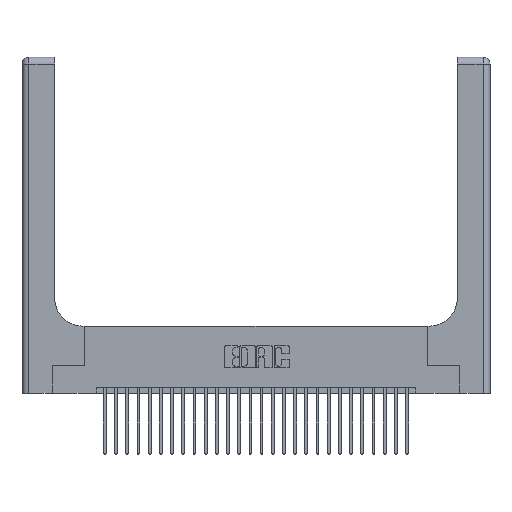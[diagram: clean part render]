
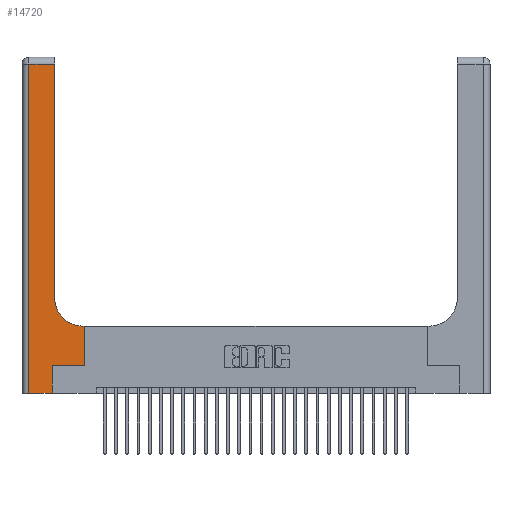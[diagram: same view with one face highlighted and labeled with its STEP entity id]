
A CAD part, top view. The second image highlights one B-rep face of the part: STEP entity #14720.
In plain terms, the highlighted planar face has unit normal (0, 0, 1).
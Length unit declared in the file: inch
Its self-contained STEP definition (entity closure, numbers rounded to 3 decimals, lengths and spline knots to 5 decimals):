
#814 = EDGE_CURVE ( 'NONE', #4730, #16422, #15518, .T. ) ;
#1194 = ORIENTED_EDGE ( 'NONE', *, *, #24007, .T. ) ;
#1438 = VERTEX_POINT ( 'NONE', #7639 ) ;
#1827 = VECTOR ( 'NONE', #13292, 39.37008 ) ;
#3280 = VECTOR ( 'NONE', #25573, 39.37008 ) ;
#4053 = VECTOR ( 'NONE', #12388, 39.37008 ) ;
#4461 = CARTESIAN_POINT ( 'NONE',  ( 0.06, 3., 0.37 ) ) ;
#4730 = VERTEX_POINT ( 'NONE', #5925 ) ;
#4941 = CARTESIAN_POINT ( 'NONE',  ( 0.06, 0., 0.37 ) ) ;
#5925 = CARTESIAN_POINT ( 'NONE',  ( 0.269, 0., 0.37 ) ) ;
#5981 = CIRCLE ( 'NONE', #23748, 0.25 ) ;
#6549 = LINE ( 'NONE', #12526, #28282 ) ;
#7168 = DIRECTION ( 'NONE',  ( 0., 0., -1. ) ) ;
#7337 = CARTESIAN_POINT ( 'NONE',  ( 0.2915, 2.94, 0.37 ) ) ;
#7361 = PLANE ( 'NONE',  #12674 ) ;
#7451 = VERTEX_POINT ( 'NONE', #16705 ) ;
#7639 = CARTESIAN_POINT ( 'NONE',  ( 0.06, 2.94, 0.37 ) ) ;
#8438 = ORIENTED_EDGE ( 'NONE', *, *, #15422, .T. ) ;
#8717 = CARTESIAN_POINT ( 'NONE',  ( 0.5415, 0.6, 0.37 ) ) ;
#10127 = CARTESIAN_POINT ( 'NONE',  ( 0.5585, 0.25, 0.37 ) ) ;
#10385 = CARTESIAN_POINT ( 'NONE',  ( 0.2915, 0.6, 0.37 ) ) ;
#10492 = CARTESIAN_POINT ( 'NONE',  ( 0.5585, 0.25, 0.37 ) ) ;
#11010 = CARTESIAN_POINT ( 'NONE',  ( 0.269, 0.25, 0.37 ) ) ;
#11692 = LINE ( 'NONE', #4461, #16961 ) ;
#11914 = CARTESIAN_POINT ( 'NONE',  ( 0., 3., 0.37 ) ) ;
#12181 = CARTESIAN_POINT ( 'NONE',  ( 0., 0., 0.37 ) ) ;
#12295 = VERTEX_POINT ( 'NONE', #8717 ) ;
#12388 = DIRECTION ( 'NONE',  ( 0., 1., 0. ) ) ;
#12506 = ORIENTED_EDGE ( 'NONE', *, *, #28689, .T. ) ;
#12526 = CARTESIAN_POINT ( 'NONE',  ( 0.2915, 3., 0.37 ) ) ;
#12674 = AXIS2_PLACEMENT_3D ( 'NONE', #11914, #27552, #14192 ) ;
#13132 = VERTEX_POINT ( 'NONE', #7337 ) ;
#13292 = DIRECTION ( 'NONE',  ( 1., 0., 0. ) ) ;
#13772 = ORIENTED_EDGE ( 'NONE', *, *, #25143, .T. ) ;
#13890 = LINE ( 'NONE', #12181, #3280 ) ;
#13974 = VERTEX_POINT ( 'NONE', #10492 ) ;
#14155 = CARTESIAN_POINT ( 'NONE',  ( 0., 2.94, 0.37 ) ) ;
#14192 = DIRECTION ( 'NONE',  ( -1., 0., 0. ) ) ;
#14537 = LINE ( 'NONE', #11010, #1827 ) ;
#14594 = LINE ( 'NONE', #14155, #25773 ) ;
#14720 = ADVANCED_FACE ( 'NONE', ( #25456 ), #7361, .F. ) ;
#14789 = DIRECTION ( 'NONE',  ( 0., 1., 0. ) ) ;
#15374 = EDGE_CURVE ( 'NONE', #13132, #1438, #14594, .T. ) ;
#15384 = VERTEX_POINT ( 'NONE', #23232 ) ;
#15422 = EDGE_CURVE ( 'NONE', #18927, #4730, #13890, .T. ) ;
#15518 = LINE ( 'NONE', #16725, #27376 ) ;
#16422 = VERTEX_POINT ( 'NONE', #17893 ) ;
#16705 = CARTESIAN_POINT ( 'NONE',  ( 0.2915, 0.85, 0.37 ) ) ;
#16725 = CARTESIAN_POINT ( 'NONE',  ( 0.269, 0., 0.37 ) ) ;
#16821 = ORIENTED_EDGE ( 'NONE', *, *, #15374, .T. ) ;
#16917 = ORIENTED_EDGE ( 'NONE', *, *, #27693, .T. ) ;
#16961 = VECTOR ( 'NONE', #17948, 39.37008 ) ;
#17143 = DIRECTION ( 'NONE',  ( -1., 0., 0. ) ) ;
#17893 = CARTESIAN_POINT ( 'NONE',  ( 0.269, 0.25, 0.37 ) ) ;
#17948 = DIRECTION ( 'NONE',  ( 0., -1., 0. ) ) ;
#18627 = DIRECTION ( 'NONE',  ( -1., 0., 0. ) ) ;
#18927 = VERTEX_POINT ( 'NONE', #4941 ) ;
#20297 = VECTOR ( 'NONE', #17143, 39.37008 ) ;
#20626 = CARTESIAN_POINT ( 'NONE',  ( 0.5415, 0.85, 0.37 ) ) ;
#21302 = ORIENTED_EDGE ( 'NONE', *, *, #26516, .T. ) ;
#21704 = LINE ( 'NONE', #10385, #20297 ) ;
#22689 = LINE ( 'NONE', #10127, #4053 ) ;
#22880 = DIRECTION ( 'NONE',  ( 1., 0., 0. ) ) ;
#23232 = CARTESIAN_POINT ( 'NONE',  ( 0.5585, 0.6, 0.37 ) ) ;
#23383 = DIRECTION ( 'NONE',  ( 0., 1., 0. ) ) ;
#23619 = ORIENTED_EDGE ( 'NONE', *, *, #814, .T. ) ;
#23748 = AXIS2_PLACEMENT_3D ( 'NONE', #20626, #7168, #22880 ) ;
#23944 = EDGE_CURVE ( 'NONE', #16422, #13974, #14537, .T. ) ;
#24007 = EDGE_CURVE ( 'NONE', #1438, #18927, #11692, .T. ) ;
#25143 = EDGE_CURVE ( 'NONE', #12295, #7451, #5981, .T. ) ;
#25456 = FACE_OUTER_BOUND ( 'NONE', #27937, .T. ) ;
#25573 = DIRECTION ( 'NONE',  ( 1., 0., 0. ) ) ;
#25773 = VECTOR ( 'NONE', #18627, 39.37008 ) ;
#26516 = EDGE_CURVE ( 'NONE', #15384, #12295, #21704, .T. ) ;
#27376 = VECTOR ( 'NONE', #23383, 39.37008 ) ;
#27552 = DIRECTION ( 'NONE',  ( 0., 0., -1. ) ) ;
#27693 = EDGE_CURVE ( 'NONE', #13974, #15384, #22689, .T. ) ;
#27937 = EDGE_LOOP ( 'NONE', ( #12506, #16821, #1194, #8438, #23619, #28897, #16917, #21302, #13772 ) ) ;
#28282 = VECTOR ( 'NONE', #14789, 39.37008 ) ;
#28689 = EDGE_CURVE ( 'NONE', #7451, #13132, #6549, .T. ) ;
#28897 = ORIENTED_EDGE ( 'NONE', *, *, #23944, .T. ) ;
